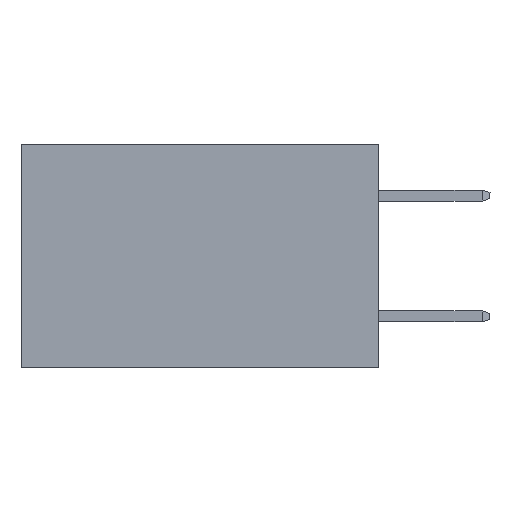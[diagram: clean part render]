
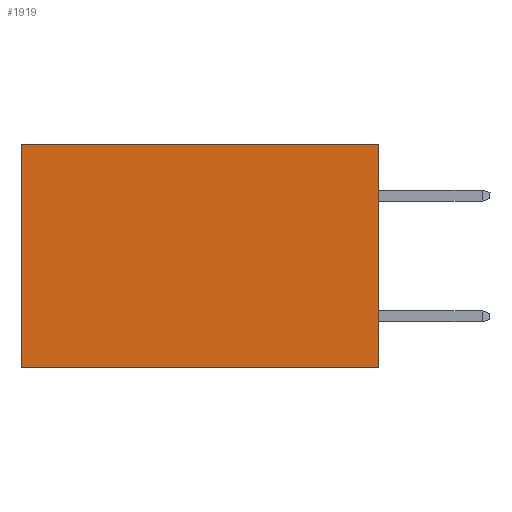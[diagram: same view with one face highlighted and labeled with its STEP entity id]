
A CAD part, left-side view. The second image highlights one B-rep face of the part: STEP entity #1919.
In plain terms, the highlighted planar face has unit normal (-1, 0, 0).
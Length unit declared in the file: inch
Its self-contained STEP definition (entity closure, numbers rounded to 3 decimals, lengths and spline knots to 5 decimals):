
#240 = VECTOR ( 'NONE', #4900, 39.37008 ) ;
#369 = VERTEX_POINT ( 'NONE', #2914 ) ;
#971 = VECTOR ( 'NONE', #4608, 39.37008 ) ;
#1314 = AXIS2_PLACEMENT_3D ( 'NONE', #7801, #2583, #4058 ) ;
#1347 = EDGE_LOOP ( 'NONE', ( #7072, #7843, #2053, #8504 ) ) ;
#1445 = CARTESIAN_POINT ( 'NONE',  ( 0.277, 0., 0. ) ) ;
#1511 = EDGE_CURVE ( 'NONE', #2297, #369, #5873, .T. ) ;
#1919 = ADVANCED_FACE ( 'NONE', ( #4692 ), #8519, .F. ) ;
#2053 = ORIENTED_EDGE ( 'NONE', *, *, #4387, .F. ) ;
#2297 = VERTEX_POINT ( 'NONE', #1445 ) ;
#2583 = DIRECTION ( 'NONE',  ( 1., 0., 0. ) ) ;
#2914 = CARTESIAN_POINT ( 'NONE',  ( 0.277, 0.59, 0. ) ) ;
#3268 = CARTESIAN_POINT ( 'NONE',  ( 0.277, 0., -0.37 ) ) ;
#3627 = LINE ( 'NONE', #3268, #7091 ) ;
#3843 = CARTESIAN_POINT ( 'NONE',  ( 0.277, 0.59, -0.37 ) ) ;
#4057 = DIRECTION ( 'NONE',  ( 0., 0., -1. ) ) ;
#4058 = DIRECTION ( 'NONE',  ( 0., 0., -1. ) ) ;
#4387 = EDGE_CURVE ( 'NONE', #2297, #7492, #4728, .T. ) ;
#4513 = LINE ( 'NONE', #5768, #7338 ) ;
#4524 = CARTESIAN_POINT ( 'NONE',  ( 0.277, 0., -0.37 ) ) ;
#4608 = DIRECTION ( 'NONE',  ( 0., 0., -1. ) ) ;
#4692 = FACE_OUTER_BOUND ( 'NONE', #1347, .T. ) ;
#4728 = LINE ( 'NONE', #4524, #971 ) ;
#4900 = DIRECTION ( 'NONE',  ( 0., 1., 0. ) ) ;
#4977 = EDGE_CURVE ( 'NONE', #369, #6791, #4513, .T. ) ;
#5768 = CARTESIAN_POINT ( 'NONE',  ( 0.277, 0.59, -0.37 ) ) ;
#5873 = LINE ( 'NONE', #7925, #240 ) ;
#5926 = DIRECTION ( 'NONE',  ( 0., 1., 0. ) ) ;
#6791 = VERTEX_POINT ( 'NONE', #3843 ) ;
#7072 = ORIENTED_EDGE ( 'NONE', *, *, #4977, .T. ) ;
#7091 = VECTOR ( 'NONE', #5926, 39.37008 ) ;
#7338 = VECTOR ( 'NONE', #4057, 39.37008 ) ;
#7492 = VERTEX_POINT ( 'NONE', #7748 ) ;
#7748 = CARTESIAN_POINT ( 'NONE',  ( 0.277, 0., -0.37 ) ) ;
#7801 = CARTESIAN_POINT ( 'NONE',  ( 0.277, 0., -0.37 ) ) ;
#7843 = ORIENTED_EDGE ( 'NONE', *, *, #8691, .F. ) ;
#7925 = CARTESIAN_POINT ( 'NONE',  ( 0.277, 0., 0. ) ) ;
#8504 = ORIENTED_EDGE ( 'NONE', *, *, #1511, .T. ) ;
#8519 = PLANE ( 'NONE',  #1314 ) ;
#8691 = EDGE_CURVE ( 'NONE', #7492, #6791, #3627, .T. ) ;
